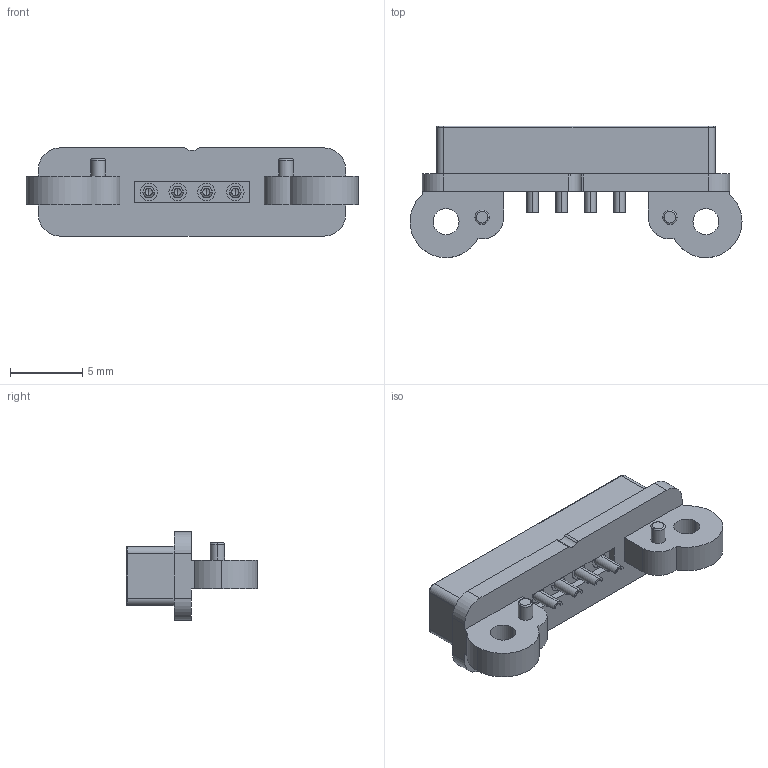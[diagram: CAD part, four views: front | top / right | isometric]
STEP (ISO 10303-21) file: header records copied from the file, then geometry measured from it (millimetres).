
FILE_DESCRIPTION (( 'STEP AP214' ), '1' );
FILE_NAME ('686J0421450124E.STEP', '2023-08-15T17:15:11', ( '' ), ( '' ), 'SwSTEP 2.0', 'SolidWorks 2023', '' );
FILE_SCHEMA (( 'AUTOMOTIVE_DESIGN' ));
Length unit declared in the file: millimetre
Products named in the file (1): 686J0421450124E
Bounding box: 23 x 9.09 x 6.1 mm (x, y, z)
Volume: 475.5 mm3; surface area: 678 mm2
Topology: 5 solids, 5 shells, 203 faces, 500 edges, 320 vertices
Faces by surface type: plane 78, cylinder 76, torus 20, cone 16, bspline 13
Entity records: 6755 total; most frequent: CARTESIAN_POINT 1869, DIRECTION 1032, ORIENTED_EDGE 984, EDGE_CURVE 492, AXIS2_PLACEMENT_3D 391, VERTEX_POINT 320, LINE 250, VECTOR 250
